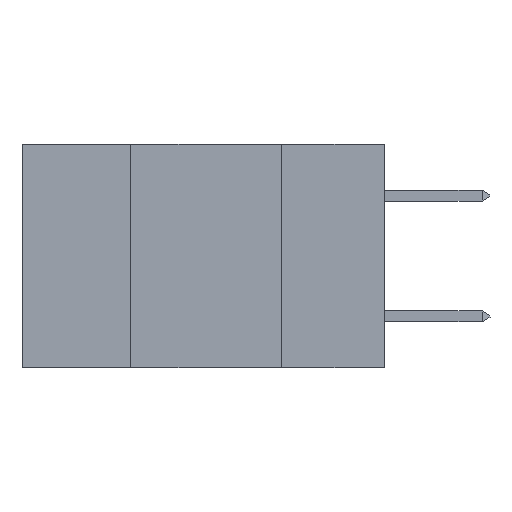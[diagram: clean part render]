
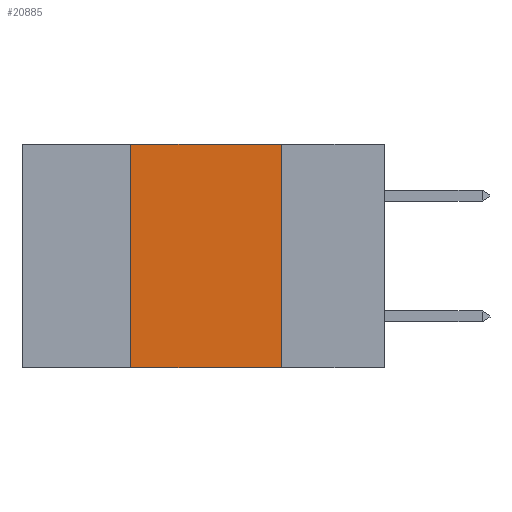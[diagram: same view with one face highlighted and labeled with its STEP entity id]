
A CAD part, left-side view. The second image highlights one B-rep face of the part: STEP entity #20885.
In plain terms, the highlighted planar face has unit normal (-1, 0, 0).
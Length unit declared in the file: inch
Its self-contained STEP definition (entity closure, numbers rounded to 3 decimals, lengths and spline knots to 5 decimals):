
#2067 = CARTESIAN_POINT ( 'NONE',  ( 0., 0.17, 0. ) ) ;
#3871 = FACE_OUTER_BOUND ( 'NONE', #4869, .T. ) ;
#4108 = EDGE_CURVE ( 'NONE', #9926, #17055, #12422, .T. ) ;
#4869 = EDGE_LOOP ( 'NONE', ( #5969, #8615, #13654, #16062 ) ) ;
#5579 = CARTESIAN_POINT ( 'NONE',  ( 0., 0.42, 0. ) ) ;
#5827 = LINE ( 'NONE', #19187, #10009 ) ;
#5969 = ORIENTED_EDGE ( 'NONE', *, *, #8946, .F. ) ;
#6462 = VERTEX_POINT ( 'NONE', #2067 ) ;
#6652 = DIRECTION ( 'NONE',  ( 1., 0., 0. ) ) ;
#6765 = VECTOR ( 'NONE', #17663, 39.37008 ) ;
#6769 = CARTESIAN_POINT ( 'NONE',  ( 0., 0.42, 0. ) ) ;
#8615 = ORIENTED_EDGE ( 'NONE', *, *, #11505, .F. ) ;
#8647 = CARTESIAN_POINT ( 'NONE',  ( 0., 0.17, -0.37 ) ) ;
#8946 = EDGE_CURVE ( 'NONE', #6462, #17055, #5827, .T. ) ;
#9624 = LINE ( 'NONE', #14073, #23351 ) ;
#9926 = VERTEX_POINT ( 'NONE', #11666 ) ;
#10009 = VECTOR ( 'NONE', #17439, 39.37008 ) ;
#11505 = EDGE_CURVE ( 'NONE', #21598, #6462, #9624, .T. ) ;
#11666 = CARTESIAN_POINT ( 'NONE',  ( 0., 0.42, -0.37 ) ) ;
#12422 = LINE ( 'NONE', #19778, #20888 ) ;
#13654 = ORIENTED_EDGE ( 'NONE', *, *, #13841, .F. ) ;
#13823 = PLANE ( 'NONE',  #19548 ) ;
#13841 = EDGE_CURVE ( 'NONE', #9926, #21598, #16960, .T. ) ;
#14073 = CARTESIAN_POINT ( 'NONE',  ( 0., 0.6, 0. ) ) ;
#16062 = ORIENTED_EDGE ( 'NONE', *, *, #4108, .T. ) ;
#16204 = DIRECTION ( 'NONE',  ( 0., -1., 0. ) ) ;
#16960 = LINE ( 'NONE', #6769, #6765 ) ;
#17055 = VERTEX_POINT ( 'NONE', #8647 ) ;
#17439 = DIRECTION ( 'NONE',  ( 0., 0., -1. ) ) ;
#17472 = CARTESIAN_POINT ( 'NONE',  ( 0., 0.6, 0. ) ) ;
#17663 = DIRECTION ( 'NONE',  ( 0., 0., 1. ) ) ;
#19187 = CARTESIAN_POINT ( 'NONE',  ( 0., 0.17, 0. ) ) ;
#19288 = DIRECTION ( 'NONE',  ( 0., 0., -1. ) ) ;
#19548 = AXIS2_PLACEMENT_3D ( 'NONE', #17472, #6652, #19288 ) ;
#19778 = CARTESIAN_POINT ( 'NONE',  ( 0., 0.6, -0.37 ) ) ;
#20885 = ADVANCED_FACE ( 'NONE', ( #3871 ), #13823, .F. ) ;
#20888 = VECTOR ( 'NONE', #16204, 39.37008 ) ;
#21598 = VERTEX_POINT ( 'NONE', #5579 ) ;
#22954 = DIRECTION ( 'NONE',  ( 0., -1., 0. ) ) ;
#23351 = VECTOR ( 'NONE', #22954, 39.37008 ) ;
